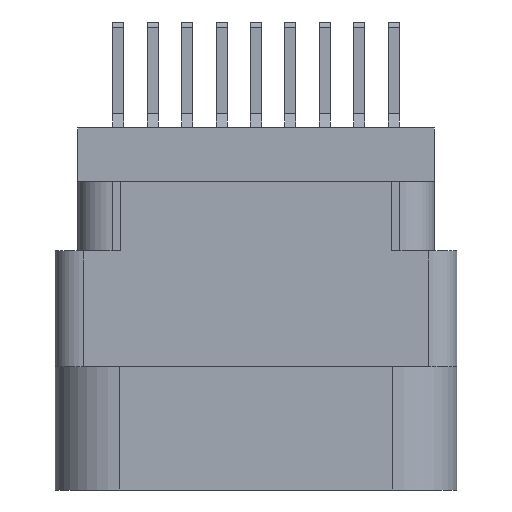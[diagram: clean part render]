
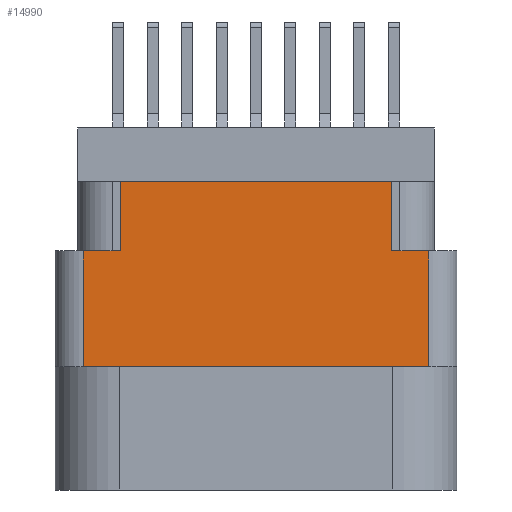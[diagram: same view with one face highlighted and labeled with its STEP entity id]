
A CAD part, left-side view. The second image highlights one B-rep face of the part: STEP entity #14990.
In plain terms, the highlighted planar face has unit normal (-1, 0, 0).
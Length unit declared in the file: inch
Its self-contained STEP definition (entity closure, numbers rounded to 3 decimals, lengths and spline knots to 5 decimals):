
#1507 = CARTESIAN_POINT ( 'NONE',  ( -1., -0.376, -0.268 ) ) ;
#2911 = ORIENTED_EDGE ( 'NONE', *, *, #31126, .T. ) ;
#2961 = CARTESIAN_POINT ( 'NONE',  ( -1., 0.376, -0.268 ) ) ;
#3145 = EDGE_CURVE ( 'NONE', #6858, #6329, #31158, .T. ) ;
#5223 = VERTEX_POINT ( 'NONE', #24209 ) ;
#5478 = LINE ( 'NONE', #7927, #31083 ) ;
#5988 = LINE ( 'NONE', #15115, #21410 ) ;
#6329 = VERTEX_POINT ( 'NONE', #30073 ) ;
#6858 = VERTEX_POINT ( 'NONE', #28064 ) ;
#7092 = LINE ( 'NONE', #30074, #9912 ) ;
#7927 = CARTESIAN_POINT ( 'NONE',  ( -1., 0., -0.268 ) ) ;
#8764 = VECTOR ( 'NONE', #23344, 39.37008 ) ;
#9384 = ORIENTED_EDGE ( 'NONE', *, *, #20916, .F. ) ;
#9498 = DIRECTION ( 'NONE',  ( 0., -1., 0. ) ) ;
#9684 = EDGE_CURVE ( 'NONE', #16365, #9808, #10040, .T. ) ;
#9808 = VERTEX_POINT ( 'NONE', #1507 ) ;
#9912 = VECTOR ( 'NONE', #9498, 39.37008 ) ;
#9970 = ORIENTED_EDGE ( 'NONE', *, *, #22495, .F. ) ;
#10040 = LINE ( 'NONE', #16363, #12497 ) ;
#10553 = ORIENTED_EDGE ( 'NONE', *, *, #9684, .F. ) ;
#10955 = CARTESIAN_POINT ( 'NONE',  ( -1., -0.376, -0.52 ) ) ;
#11340 = DIRECTION ( 'NONE',  ( -1., 0., 0. ) ) ;
#11832 = VERTEX_POINT ( 'NONE', #2961 ) ;
#12244 = FACE_OUTER_BOUND ( 'NONE', #27919, .T. ) ;
#12497 = VECTOR ( 'NONE', #18978, 39.37008 ) ;
#14990 = ADVANCED_FACE ( 'NONE', ( #12244 ), #21443, .T. ) ;
#15115 = CARTESIAN_POINT ( 'NONE',  ( -1., -0.296, -0.268 ) ) ;
#15780 = LINE ( 'NONE', #25881, #19454 ) ;
#16363 = CARTESIAN_POINT ( 'NONE',  ( -1., 0., -0.268 ) ) ;
#16365 = VERTEX_POINT ( 'NONE', #33196 ) ;
#16638 = ORIENTED_EDGE ( 'NONE', *, *, #19326, .T. ) ;
#17331 = VERTEX_POINT ( 'NONE', #23138 ) ;
#18664 = VERTEX_POINT ( 'NONE', #10955 ) ;
#18978 = DIRECTION ( 'NONE',  ( 0., -1., 0. ) ) ;
#19248 = VECTOR ( 'NONE', #24809, 39.37008 ) ;
#19326 = EDGE_CURVE ( 'NONE', #5223, #18664, #7092, .T. ) ;
#19454 = VECTOR ( 'NONE', #20895, 39.37008 ) ;
#20718 = CARTESIAN_POINT ( 'NONE',  ( -1., 0.296, -0.268 ) ) ;
#20895 = DIRECTION ( 'NONE',  ( 0., 0., 1. ) ) ;
#20916 = EDGE_CURVE ( 'NONE', #6329, #17331, #32157, .T. ) ;
#21410 = VECTOR ( 'NONE', #30687, 39.37008 ) ;
#21443 = PLANE ( 'NONE',  #26126 ) ;
#21551 = DIRECTION ( 'NONE',  ( 0., 0., 1. ) ) ;
#22495 = EDGE_CURVE ( 'NONE', #11832, #6858, #5478, .T. ) ;
#23138 = CARTESIAN_POINT ( 'NONE',  ( -1., -0.296, -0.117 ) ) ;
#23205 = VECTOR ( 'NONE', #27394, 39.37008 ) ;
#23344 = DIRECTION ( 'NONE',  ( 0., 0., 1. ) ) ;
#24070 = CARTESIAN_POINT ( 'NONE',  ( -1., -0.438, -0.789 ) ) ;
#24122 = ORIENTED_EDGE ( 'NONE', *, *, #3145, .F. ) ;
#24209 = CARTESIAN_POINT ( 'NONE',  ( -1., 0.376, -0.52 ) ) ;
#24809 = DIRECTION ( 'NONE',  ( 0., 0., -1. ) ) ;
#25240 = EDGE_CURVE ( 'NONE', #16365, #17331, #5988, .T. ) ;
#25881 = CARTESIAN_POINT ( 'NONE',  ( -1., -0.376, -0.789 ) ) ;
#26084 = DIRECTION ( 'NONE',  ( 0., -1., 0. ) ) ;
#26126 = AXIS2_PLACEMENT_3D ( 'NONE', #24070, #11340, #21551 ) ;
#27394 = DIRECTION ( 'NONE',  ( 0., -1., 0. ) ) ;
#27919 = EDGE_LOOP ( 'NONE', ( #9970, #2911, #16638, #28312, #10553, #32614, #9384, #24122 ) ) ;
#28064 = CARTESIAN_POINT ( 'NONE',  ( -1., 0.296, -0.268 ) ) ;
#28312 = ORIENTED_EDGE ( 'NONE', *, *, #32628, .T. ) ;
#30073 = CARTESIAN_POINT ( 'NONE',  ( -1., 0.296, -0.117 ) ) ;
#30074 = CARTESIAN_POINT ( 'NONE',  ( -1., 0., -0.52 ) ) ;
#30230 = CARTESIAN_POINT ( 'NONE',  ( -1., 0.438, -0.117 ) ) ;
#30687 = DIRECTION ( 'NONE',  ( 0., 0., 1. ) ) ;
#31083 = VECTOR ( 'NONE', #26084, 39.37008 ) ;
#31126 = EDGE_CURVE ( 'NONE', #11832, #5223, #32710, .T. ) ;
#31158 = LINE ( 'NONE', #20718, #8764 ) ;
#32157 = LINE ( 'NONE', #30230, #23205 ) ;
#32444 = CARTESIAN_POINT ( 'NONE',  ( -1., 0.376, -0.789 ) ) ;
#32614 = ORIENTED_EDGE ( 'NONE', *, *, #25240, .T. ) ;
#32628 = EDGE_CURVE ( 'NONE', #18664, #9808, #15780, .T. ) ;
#32710 = LINE ( 'NONE', #32444, #19248 ) ;
#33196 = CARTESIAN_POINT ( 'NONE',  ( -1., -0.296, -0.268 ) ) ;
